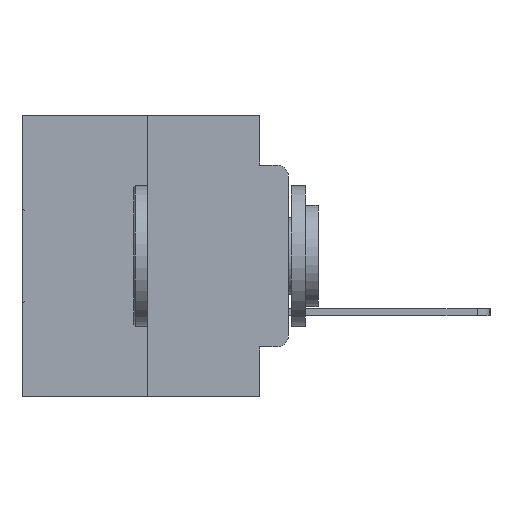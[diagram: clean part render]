
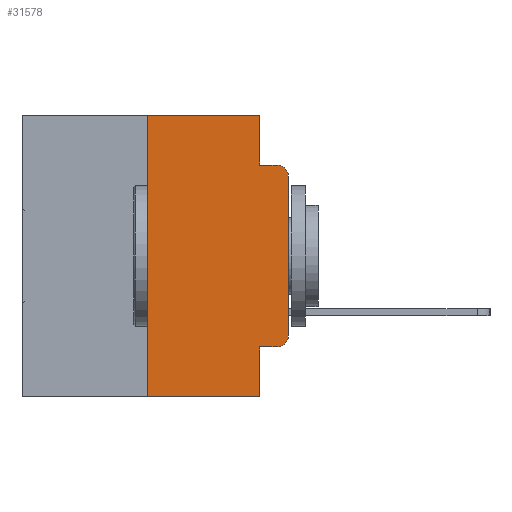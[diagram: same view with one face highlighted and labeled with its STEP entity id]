
A CAD part, left-side view. The second image highlights one B-rep face of the part: STEP entity #31578.
In plain terms, the highlighted planar face has unit normal (-1, 0, 0).
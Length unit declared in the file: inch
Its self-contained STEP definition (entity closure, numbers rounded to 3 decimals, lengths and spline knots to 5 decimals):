
#211 = EDGE_CURVE ( 'NONE', #10278, #24993, #1072, .T. ) ;
#623 = ORIENTED_EDGE ( 'NONE', *, *, #30380, .F. ) ;
#1072 = LINE ( 'NONE', #30607, #19075 ) ;
#1113 = CARTESIAN_POINT ( 'NONE',  ( 0., 0.473, -0.5 ) ) ;
#1720 = CARTESIAN_POINT ( 'NONE',  ( 0., 0.25, 0. ) ) ;
#2454 = CARTESIAN_POINT ( 'NONE',  ( 0., 0.02, -0.1085 ) ) ;
#2656 = EDGE_CURVE ( 'NONE', #24993, #24994, #14743, .T. ) ;
#3112 = EDGE_CURVE ( 'NONE', #3629, #30748, #23899, .T. ) ;
#3629 = VERTEX_POINT ( 'NONE', #16039 ) ;
#3849 = CARTESIAN_POINT ( 'NONE',  ( 0., 0.473, 0. ) ) ;
#4017 = VECTOR ( 'NONE', #13421, 39.37008 ) ;
#4185 = DIRECTION ( 'NONE',  ( 0., 0., 1. ) ) ;
#4483 = VECTOR ( 'NONE', #7685, 39.37008 ) ;
#4488 = ORIENTED_EDGE ( 'NONE', *, *, #20394, .F. ) ;
#4784 = LINE ( 'NONE', #1113, #4017 ) ;
#4909 = DIRECTION ( 'NONE',  ( 0., 0., -1. ) ) ;
#5293 = VECTOR ( 'NONE', #21016, 39.37008 ) ;
#5294 = DIRECTION ( 'NONE',  ( -1., 0., 0. ) ) ;
#5659 = AXIS2_PLACEMENT_3D ( 'NONE', #2454, #19582, #4909 ) ;
#5977 = VECTOR ( 'NONE', #4185, 39.37008 ) ;
#6218 = EDGE_CURVE ( 'NONE', #12715, #23020, #26064, .T. ) ;
#6661 = CARTESIAN_POINT ( 'NONE',  ( 0., 0., 0. ) ) ;
#6905 = VERTEX_POINT ( 'NONE', #9997 ) ;
#7167 = EDGE_CURVE ( 'NONE', #10278, #10737, #13008, .T. ) ;
#7608 = DIRECTION ( 'NONE',  ( 1., 0., 0. ) ) ;
#7685 = DIRECTION ( 'NONE',  ( 0., -1., 0. ) ) ;
#9092 = EDGE_CURVE ( 'NONE', #24994, #12715, #12490, .T. ) ;
#9122 = DIRECTION ( 'NONE',  ( 0., 0., 1. ) ) ;
#9344 = CARTESIAN_POINT ( 'NONE',  ( 0., 0.051, 0. ) ) ;
#9575 = DIRECTION ( 'NONE',  ( 0., 0., -1. ) ) ;
#9997 = CARTESIAN_POINT ( 'NONE',  ( 0., 0.25, 0. ) ) ;
#10278 = VERTEX_POINT ( 'NONE', #23057 ) ;
#10290 = AXIS2_PLACEMENT_3D ( 'NONE', #14045, #5294, #11805 ) ;
#10737 = VERTEX_POINT ( 'NONE', #15164 ) ;
#11468 = EDGE_CURVE ( 'NONE', #16511, #10737, #4784, .T. ) ;
#11644 = VECTOR ( 'NONE', #9575, 39.37008 ) ;
#11782 = LINE ( 'NONE', #19896, #4483 ) ;
#11805 = DIRECTION ( 'NONE',  ( 0., 0., -1. ) ) ;
#12215 = ORIENTED_EDGE ( 'NONE', *, *, #11468, .T. ) ;
#12490 = LINE ( 'NONE', #6661, #5977 ) ;
#12715 = VERTEX_POINT ( 'NONE', #19675 ) ;
#13008 = LINE ( 'NONE', #18335, #17984 ) ;
#13201 = DIRECTION ( 'NONE',  ( 0., 0., -1. ) ) ;
#13421 = DIRECTION ( 'NONE',  ( 0., -1., 0. ) ) ;
#14045 = CARTESIAN_POINT ( 'NONE',  ( 0., 0.02, -0.3915 ) ) ;
#14070 = CARTESIAN_POINT ( 'NONE',  ( 0., 0.051, -0.0885 ) ) ;
#14743 = CIRCLE ( 'NONE', #10290, 0.02 ) ;
#15164 = CARTESIAN_POINT ( 'NONE',  ( 0., 0.051, -0.5 ) ) ;
#15317 = ORIENTED_EDGE ( 'NONE', *, *, #2656, .T. ) ;
#15604 = EDGE_CURVE ( 'NONE', #16511, #6905, #30561, .T. ) ;
#15961 = ORIENTED_EDGE ( 'NONE', *, *, #3112, .F. ) ;
#16039 = CARTESIAN_POINT ( 'NONE',  ( 0., 0.051, 0. ) ) ;
#16420 = EDGE_LOOP ( 'NONE', ( #28918, #27032, #623, #15961, #4488, #22978, #12215, #22605, #16451, #15317 ) ) ;
#16451 = ORIENTED_EDGE ( 'NONE', *, *, #211, .T. ) ;
#16511 = VERTEX_POINT ( 'NONE', #20110 ) ;
#17984 = VECTOR ( 'NONE', #13201, 39.37008 ) ;
#18316 = LINE ( 'NONE', #3849, #5293 ) ;
#18335 = CARTESIAN_POINT ( 'NONE',  ( 0., 0.051, 0. ) ) ;
#19075 = VECTOR ( 'NONE', #27804, 39.37008 ) ;
#19582 = DIRECTION ( 'NONE',  ( -1., 0., 0. ) ) ;
#19675 = CARTESIAN_POINT ( 'NONE',  ( 0., 0., -0.1085 ) ) ;
#19896 = CARTESIAN_POINT ( 'NONE',  ( 0., 0.051, -0.0885 ) ) ;
#20110 = CARTESIAN_POINT ( 'NONE',  ( 0., 0.25, -0.5 ) ) ;
#20394 = EDGE_CURVE ( 'NONE', #6905, #3629, #18316, .T. ) ;
#20932 = CARTESIAN_POINT ( 'NONE',  ( 0., 0.02, -0.4115 ) ) ;
#21016 = DIRECTION ( 'NONE',  ( 0., -1., 0. ) ) ;
#22297 = CARTESIAN_POINT ( 'NONE',  ( 0., 0.473, 0. ) ) ;
#22393 = CARTESIAN_POINT ( 'NONE',  ( 0., 0.02, -0.0885 ) ) ;
#22605 = ORIENTED_EDGE ( 'NONE', *, *, #7167, .F. ) ;
#22978 = ORIENTED_EDGE ( 'NONE', *, *, #15604, .F. ) ;
#23020 = VERTEX_POINT ( 'NONE', #22393 ) ;
#23057 = CARTESIAN_POINT ( 'NONE',  ( 0., 0.051, -0.4115 ) ) ;
#23306 = CARTESIAN_POINT ( 'NONE',  ( 0., 0., -0.3915 ) ) ;
#23899 = LINE ( 'NONE', #9344, #11644 ) ;
#24087 = VECTOR ( 'NONE', #9122, 39.37008 ) ;
#24723 = DIRECTION ( 'NONE',  ( 0., 0., -1. ) ) ;
#24993 = VERTEX_POINT ( 'NONE', #20932 ) ;
#24994 = VERTEX_POINT ( 'NONE', #23306 ) ;
#25482 = FACE_OUTER_BOUND ( 'NONE', #16420, .T. ) ;
#26064 = CIRCLE ( 'NONE', #5659, 0.02 ) ;
#27032 = ORIENTED_EDGE ( 'NONE', *, *, #6218, .T. ) ;
#27199 = AXIS2_PLACEMENT_3D ( 'NONE', #22297, #7608, #24723 ) ;
#27804 = DIRECTION ( 'NONE',  ( 0., -1., 0. ) ) ;
#28918 = ORIENTED_EDGE ( 'NONE', *, *, #9092, .T. ) ;
#29503 = PLANE ( 'NONE',  #27199 ) ;
#30380 = EDGE_CURVE ( 'NONE', #30748, #23020, #11782, .T. ) ;
#30561 = LINE ( 'NONE', #1720, #24087 ) ;
#30607 = CARTESIAN_POINT ( 'NONE',  ( 0., 0.051, -0.4115 ) ) ;
#30748 = VERTEX_POINT ( 'NONE', #14070 ) ;
#31578 = ADVANCED_FACE ( 'NONE', ( #25482 ), #29503, .F. ) ;
